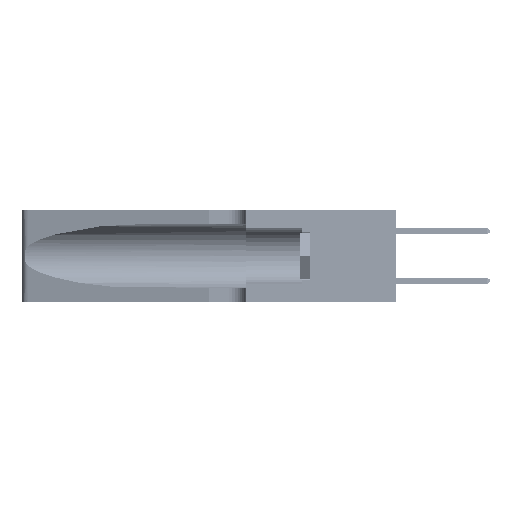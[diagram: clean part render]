
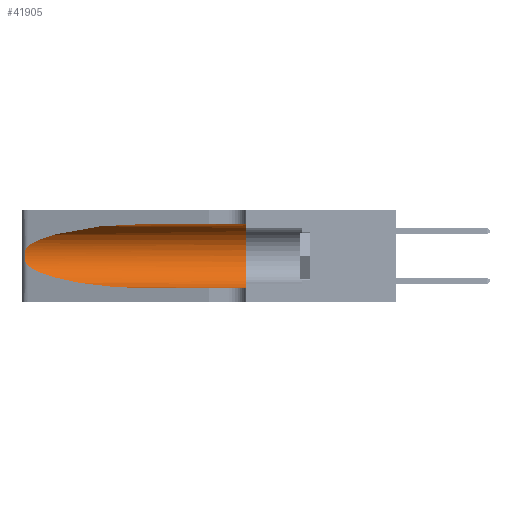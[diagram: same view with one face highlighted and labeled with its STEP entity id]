
A CAD part, left-side view. The second image highlights one B-rep face of the part: STEP entity #41905.
In plain terms, the highlighted cylindrical face has radius 3.308 mm (diameter 6.617 mm), a partial arc.
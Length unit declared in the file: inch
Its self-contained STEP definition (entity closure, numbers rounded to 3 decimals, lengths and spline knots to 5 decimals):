
#758 = VERTEX_POINT ( 'NONE', #8569 ) ;
#2427 = ORIENTED_EDGE ( 'NONE', *, *, #13576, .T. ) ;
#3013 = CARTESIAN_POINT ( 'NONE',  ( 0.25555, 1.22993, 0.14849 ) ) ;
#3113 = ORIENTED_EDGE ( 'NONE', *, *, #15284, .T. ) ;
#5127 = VERTEX_POINT ( 'NONE', #41718 ) ;
#5870 = CARTESIAN_POINT ( 'NONE',  ( 0.1305, 0.72297, 0.05475 ) ) ;
#6451 = VERTEX_POINT ( 'NONE', #5870 ) ;
#8569 = CARTESIAN_POINT ( 'NONE',  ( 0.25487, 1.22718, 0.14631 ) ) ;
#10988 = CARTESIAN_POINT ( 'NONE',  ( 0.25787, 1.23484, 0.2124 ) ) ;
#11840 = B_SPLINE_CURVE_WITH_KNOTS ( 'NONE', 3,
 ( #14800, #38503, #34719, #10988, #38671, #14979, #42632, #18952, #46568, #22917, #50501, #26911, #3013, #30887 ),
 .UNSPECIFIED., .F., .F.,
 ( 4, 2, 2, 2, 2, 2, 4 ),
 ( 0., 0.00027, 0.00053, 0.00107, 0.0016, 0.00187, 0.00214 ),
 .UNSPECIFIED. ) ;
#13576 = EDGE_CURVE ( 'NONE', #6451, #5127, #31445, .T. ) ;
#13632 = FACE_OUTER_BOUND ( 'NONE', #25965, .T. ) ;
#13920 = CARTESIAN_POINT ( 'NONE',  ( 0.1305, 0.35, 0.185 ) ) ;
#14794 = CARTESIAN_POINT ( 'NONE',  ( 0.1305, 1.61858, 0.05475 ) ) ;
#14800 = CARTESIAN_POINT ( 'NONE',  ( 0.25487, 1.22718, 0.22369 ) ) ;
#14979 = CARTESIAN_POINT ( 'NONE',  ( 0.26018, 1.23835, 0.19895 ) ) ;
#15284 = EDGE_CURVE ( 'NONE', #49628, #35878, #24838, .T. ) ;
#16988 = CARTESIAN_POINT ( 'NONE',  ( 0.1305, 0.72297, 0.05475 ) ) ;
#17090 = CARTESIAN_POINT ( 'NONE',  ( 0.18966, 0.96281, 0.31525 ) ) ;
#17364 = VECTOR ( 'NONE', #29540, 39.37008 ) ;
#17900 = DIRECTION ( 'NONE',  ( 0., 0., 1. ) ) ;
#18952 = CARTESIAN_POINT ( 'NONE',  ( 0.26075, 1.23896, 0.178 ) ) ;
#20627 = ORIENTED_EDGE ( 'NONE', *, *, #32503, .F. ) ;
#20914 = VECTOR ( 'NONE', #30707, 39.37008 ) ;
#22123 = AXIS2_PLACEMENT_3D ( 'NONE', #47765, #35909, #24136 ) ;
#22917 = CARTESIAN_POINT ( 'NONE',  ( 0.25856, 1.23593, 0.16098 ) ) ;
#23993 = EDGE_CURVE ( 'NONE', #758, #6451, #48546, .T. ) ;
#24136 = DIRECTION ( 'NONE',  ( 0., 0., -1. ) ) ;
#24838 =( BOUNDED_CURVE ( )  B_SPLINE_CURVE ( 3, ( #48840, #17090, #44906, #25220 ),
 .UNSPECIFIED., .F., .F. ) 
 B_SPLINE_CURVE_WITH_KNOTS ( ( 4, 4 ),
 ( 1.5708, 2.84003 ),
 .UNSPECIFIED. ) 
 CURVE ( )  GEOMETRIC_REPRESENTATION_ITEM ( )  RATIONAL_B_SPLINE_CURVE ( ( 1., 0.87, 0.87, 1. ) ) 
 REPRESENTATION_ITEM ( '' )  );
#25220 = CARTESIAN_POINT ( 'NONE',  ( 0.25487, 1.22718, 0.22369 ) ) ;
#25566 = CARTESIAN_POINT ( 'NONE',  ( 0.1305, 1.61858, 0.31525 ) ) ;
#25965 = EDGE_LOOP ( 'NONE', ( #3113, #35543, #29264, #2427, #20627, #41638 ) ) ;
#26911 = CARTESIAN_POINT ( 'NONE',  ( 0.25639, 1.23186, 0.15144 ) ) ;
#27082 = CARTESIAN_POINT ( 'NONE',  ( 0.25487, 1.22718, 0.22369 ) ) ;
#29264 = ORIENTED_EDGE ( 'NONE', *, *, #23993, .T. ) ;
#29540 = DIRECTION ( 'NONE',  ( 0., -1., 0. ) ) ;
#30228 = CIRCLE ( 'NONE', #46327, 0.13025 ) ;
#30707 = DIRECTION ( 'NONE',  ( 0., -1., 0. ) ) ;
#30887 = CARTESIAN_POINT ( 'NONE',  ( 0.25487, 1.22718, 0.14631 ) ) ;
#31081 = CARTESIAN_POINT ( 'NONE',  ( 0.1305, 0.72297, 0.31525 ) ) ;
#31445 = LINE ( 'NONE', #14794, #20914 ) ;
#32503 = EDGE_CURVE ( 'NONE', #35491, #5127, #30228, .T. ) ;
#32764 = CARTESIAN_POINT ( 'NONE',  ( 0.2373, 1.15595, 0.08982 ) ) ;
#32855 = CARTESIAN_POINT ( 'NONE',  ( 0.1305, 0.35, 0.31525 ) ) ;
#34719 = CARTESIAN_POINT ( 'NONE',  ( 0.25639, 1.23184, 0.21858 ) ) ;
#35491 = VERTEX_POINT ( 'NONE', #32855 ) ;
#35543 = ORIENTED_EDGE ( 'NONE', *, *, #46326, .T. ) ;
#35878 = VERTEX_POINT ( 'NONE', #27082 ) ;
#35909 = DIRECTION ( 'NONE',  ( 0., -1., 0. ) ) ;
#36733 = CARTESIAN_POINT ( 'NONE',  ( 0.25487, 1.22718, 0.14631 ) ) ;
#38419 = LINE ( 'NONE', #25566, #17364 ) ;
#38503 = CARTESIAN_POINT ( 'NONE',  ( 0.25555, 1.22994, 0.2215 ) ) ;
#38671 = CARTESIAN_POINT ( 'NONE',  ( 0.25854, 1.2359, 0.20912 ) ) ;
#40682 = CARTESIAN_POINT ( 'NONE',  ( 0.18966, 0.96281, 0.05475 ) ) ;
#41573 = DIRECTION ( 'NONE',  ( 0., 1., 0. ) ) ;
#41638 = ORIENTED_EDGE ( 'NONE', *, *, #49385, .F. ) ;
#41718 = CARTESIAN_POINT ( 'NONE',  ( 0.1305, 0.35, 0.05475 ) ) ;
#41905 = ADVANCED_FACE ( 'NONE', ( #13632 ), #43947, .F. ) ;
#42632 = CARTESIAN_POINT ( 'NONE',  ( 0.26075, 1.23896, 0.19203 ) ) ;
#43947 = CYLINDRICAL_SURFACE ( 'NONE', #22123, 0.13025 ) ;
#44906 = CARTESIAN_POINT ( 'NONE',  ( 0.2373, 1.15595, 0.28018 ) ) ;
#46326 = EDGE_CURVE ( 'NONE', #35878, #758, #11840, .T. ) ;
#46327 = AXIS2_PLACEMENT_3D ( 'NONE', #13920, #41573, #17900 ) ;
#46568 = CARTESIAN_POINT ( 'NONE',  ( 0.26017, 1.23833, 0.17102 ) ) ;
#47765 = CARTESIAN_POINT ( 'NONE',  ( 0.1305, 1.61858, 0.185 ) ) ;
#48546 =( BOUNDED_CURVE ( )  B_SPLINE_CURVE ( 3, ( #36733, #32764, #40682, #16988 ),
 .UNSPECIFIED., .F., .F. ) 
 B_SPLINE_CURVE_WITH_KNOTS ( ( 4, 4 ),
 ( 3.44316, 4.71239 ),
 .UNSPECIFIED. ) 
 CURVE ( )  GEOMETRIC_REPRESENTATION_ITEM ( )  RATIONAL_B_SPLINE_CURVE ( ( 1., 0.87, 0.87, 1. ) ) 
 REPRESENTATION_ITEM ( '' )  );
#48840 = CARTESIAN_POINT ( 'NONE',  ( 0.1305, 0.72297, 0.31525 ) ) ;
#49385 = EDGE_CURVE ( 'NONE', #49628, #35491, #38419, .T. ) ;
#49628 = VERTEX_POINT ( 'NONE', #31081 ) ;
#50501 = CARTESIAN_POINT ( 'NONE',  ( 0.25789, 1.23486, 0.15765 ) ) ;
